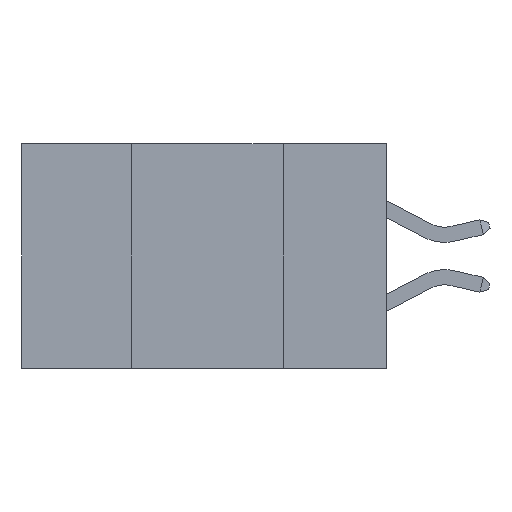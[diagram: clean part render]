
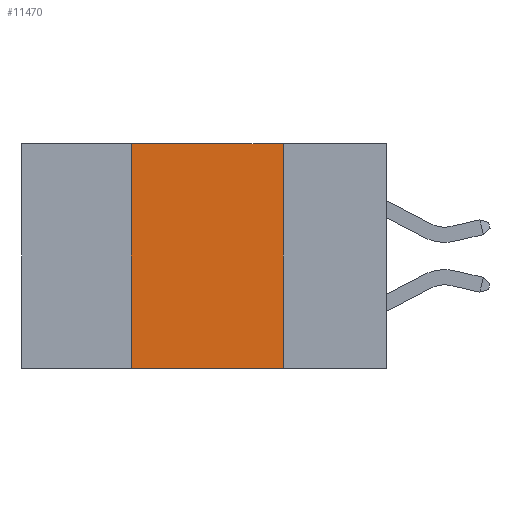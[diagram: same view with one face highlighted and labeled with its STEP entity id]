
A CAD part, left-side view. The second image highlights one B-rep face of the part: STEP entity #11470.
In plain terms, the highlighted planar face has unit normal (-1, 0, 0).
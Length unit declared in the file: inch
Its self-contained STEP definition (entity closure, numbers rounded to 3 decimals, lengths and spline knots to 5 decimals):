
#177 = EDGE_CURVE ( 'NONE', #6470, #13319, #15968, .T. ) ;
#222 = DIRECTION ( 'NONE',  ( 0., -1., 0. ) ) ;
#883 = DIRECTION ( 'NONE',  ( 1., 0., 0. ) ) ;
#1170 = CARTESIAN_POINT ( 'NONE',  ( 0., 0.6, 0. ) ) ;
#1257 = FACE_OUTER_BOUND ( 'NONE', #10745, .T. ) ;
#1709 = LINE ( 'NONE', #11935, #4779 ) ;
#2875 = DIRECTION ( 'NONE',  ( 0., -1., 0. ) ) ;
#2917 = LINE ( 'NONE', #13287, #8968 ) ;
#3781 = ORIENTED_EDGE ( 'NONE', *, *, #12491, .F. ) ;
#4779 = VECTOR ( 'NONE', #2875, 39.37008 ) ;
#6470 = VERTEX_POINT ( 'NONE', #7559 ) ;
#6678 = LINE ( 'NONE', #13647, #12774 ) ;
#7559 = CARTESIAN_POINT ( 'NONE',  ( 0., 0.42, 0. ) ) ;
#7891 = AXIS2_PLACEMENT_3D ( 'NONE', #8668, #883, #9954 ) ;
#8523 = CARTESIAN_POINT ( 'NONE',  ( 0., 0.17, 0. ) ) ;
#8668 = CARTESIAN_POINT ( 'NONE',  ( 0., 0.6, 0. ) ) ;
#8968 = VECTOR ( 'NONE', #14569, 39.37008 ) ;
#9420 = ORIENTED_EDGE ( 'NONE', *, *, #177, .F. ) ;
#9874 = CARTESIAN_POINT ( 'NONE',  ( 0., 0.42, -0.37 ) ) ;
#9896 = PLANE ( 'NONE',  #7891 ) ;
#9954 = DIRECTION ( 'NONE',  ( 0., 0., -1. ) ) ;
#10601 = EDGE_CURVE ( 'NONE', #12139, #14067, #1709, .T. ) ;
#10745 = EDGE_LOOP ( 'NONE', ( #3781, #9420, #16083, #16104 ) ) ;
#11470 = ADVANCED_FACE ( 'NONE', ( #1257 ), #9896, .F. ) ;
#11935 = CARTESIAN_POINT ( 'NONE',  ( 0., 0.6, -0.37 ) ) ;
#12139 = VERTEX_POINT ( 'NONE', #9874 ) ;
#12154 = VECTOR ( 'NONE', #222, 39.37008 ) ;
#12491 = EDGE_CURVE ( 'NONE', #13319, #14067, #2917, .T. ) ;
#12774 = VECTOR ( 'NONE', #14929, 39.37008 ) ;
#13287 = CARTESIAN_POINT ( 'NONE',  ( 0., 0.17, 0. ) ) ;
#13319 = VERTEX_POINT ( 'NONE', #8523 ) ;
#13647 = CARTESIAN_POINT ( 'NONE',  ( 0., 0.42, 0. ) ) ;
#14067 = VERTEX_POINT ( 'NONE', #15180 ) ;
#14569 = DIRECTION ( 'NONE',  ( 0., 0., -1. ) ) ;
#14650 = EDGE_CURVE ( 'NONE', #12139, #6470, #6678, .T. ) ;
#14929 = DIRECTION ( 'NONE',  ( 0., 0., 1. ) ) ;
#15180 = CARTESIAN_POINT ( 'NONE',  ( 0., 0.17, -0.37 ) ) ;
#15968 = LINE ( 'NONE', #1170, #12154 ) ;
#16083 = ORIENTED_EDGE ( 'NONE', *, *, #14650, .F. ) ;
#16104 = ORIENTED_EDGE ( 'NONE', *, *, #10601, .T. ) ;
